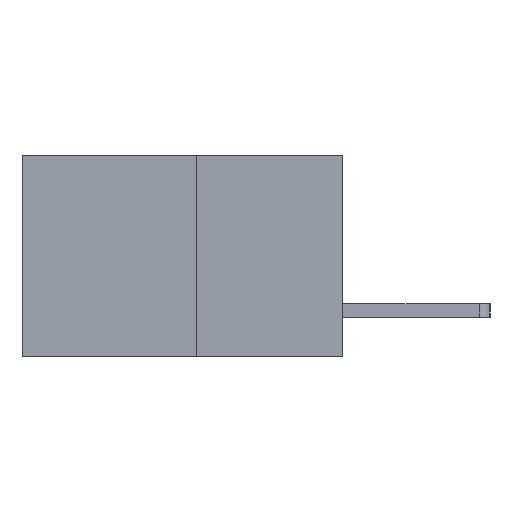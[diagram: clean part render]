
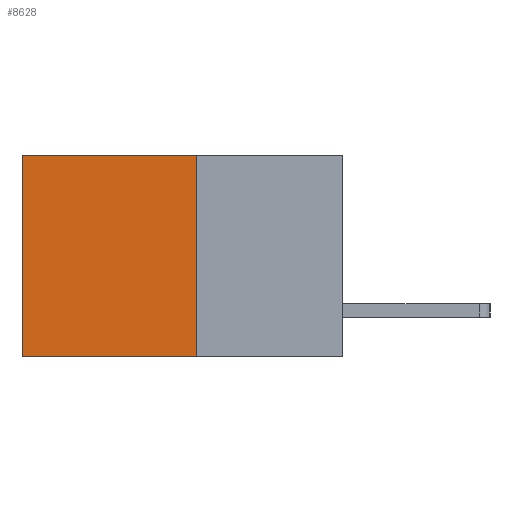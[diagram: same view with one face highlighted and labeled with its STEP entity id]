
A CAD part, left-side view. The second image highlights one B-rep face of the part: STEP entity #8628.
In plain terms, the highlighted planar face has unit normal (-1, 0, 0).
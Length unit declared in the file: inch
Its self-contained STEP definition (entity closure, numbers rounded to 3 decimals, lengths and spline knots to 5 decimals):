
#111 = VERTEX_POINT ( 'NONE', #7755 ) ;
#441 = LINE ( 'NONE', #7212, #4178 ) ;
#446 = ORIENTED_EDGE ( 'NONE', *, *, #6915, .F. ) ;
#499 = ORIENTED_EDGE ( 'NONE', *, *, #3669, .F. ) ;
#544 = AXIS2_PLACEMENT_3D ( 'NONE', #1281, #6419, #2015 ) ;
#1008 = LINE ( 'NONE', #5817, #1242 ) ;
#1016 = DIRECTION ( 'NONE',  ( 0., 1., 0. ) ) ;
#1070 = EDGE_LOOP ( 'NONE', ( #5176, #446, #499, #1102 ) ) ;
#1102 = ORIENTED_EDGE ( 'NONE', *, *, #7512, .T. ) ;
#1163 = VERTEX_POINT ( 'NONE', #5584 ) ;
#1242 = VECTOR ( 'NONE', #9091, 39.37008 ) ;
#1281 = CARTESIAN_POINT ( 'NONE',  ( 0.277, 0.27, -0.37 ) ) ;
#1303 = CARTESIAN_POINT ( 'NONE',  ( 0.277, 0.27, -0.37 ) ) ;
#2015 = DIRECTION ( 'NONE',  ( 0., 0., -1. ) ) ;
#2315 = DIRECTION ( 'NONE',  ( 0., 0., -1. ) ) ;
#2353 = CARTESIAN_POINT ( 'NONE',  ( 0.277, 0.59, -0.37 ) ) ;
#3337 = CARTESIAN_POINT ( 'NONE',  ( 0.277, 0.27, 0. ) ) ;
#3669 = EDGE_CURVE ( 'NONE', #7863, #1163, #1008, .T. ) ;
#3686 = VERTEX_POINT ( 'NONE', #7183 ) ;
#3839 = LINE ( 'NONE', #1303, #5536 ) ;
#4178 = VECTOR ( 'NONE', #7231, 39.37008 ) ;
#4986 = PLANE ( 'NONE',  #544 ) ;
#5176 = ORIENTED_EDGE ( 'NONE', *, *, #6720, .T. ) ;
#5279 = FACE_OUTER_BOUND ( 'NONE', #1070, .T. ) ;
#5536 = VECTOR ( 'NONE', #1016, 39.37008 ) ;
#5584 = CARTESIAN_POINT ( 'NONE',  ( 0.277, 0.27, -0.37 ) ) ;
#5817 = CARTESIAN_POINT ( 'NONE',  ( 0.277, 0.27, -0.37 ) ) ;
#6340 = LINE ( 'NONE', #2353, #7919 ) ;
#6419 = DIRECTION ( 'NONE',  ( 1., 0., 0. ) ) ;
#6720 = EDGE_CURVE ( 'NONE', #111, #3686, #6340, .T. ) ;
#6915 = EDGE_CURVE ( 'NONE', #1163, #3686, #3839, .T. ) ;
#7183 = CARTESIAN_POINT ( 'NONE',  ( 0.277, 0.59, -0.37 ) ) ;
#7212 = CARTESIAN_POINT ( 'NONE',  ( 0.277, 0.27, 0. ) ) ;
#7231 = DIRECTION ( 'NONE',  ( 0., 1., 0. ) ) ;
#7512 = EDGE_CURVE ( 'NONE', #7863, #111, #441, .T. ) ;
#7755 = CARTESIAN_POINT ( 'NONE',  ( 0.277, 0.59, 0. ) ) ;
#7863 = VERTEX_POINT ( 'NONE', #3337 ) ;
#7919 = VECTOR ( 'NONE', #2315, 39.37008 ) ;
#8628 = ADVANCED_FACE ( 'NONE', ( #5279 ), #4986, .F. ) ;
#9091 = DIRECTION ( 'NONE',  ( 0., 0., -1. ) ) ;
